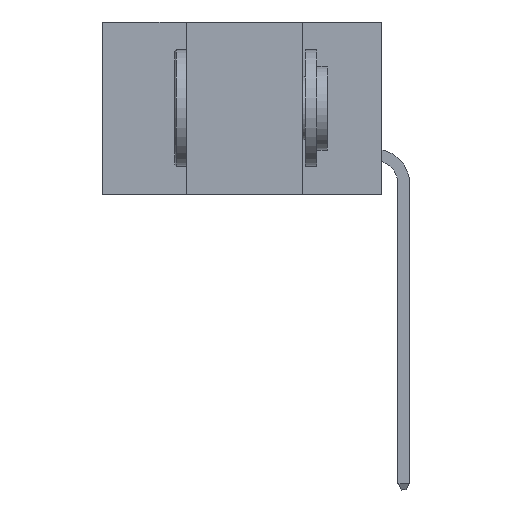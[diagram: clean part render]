
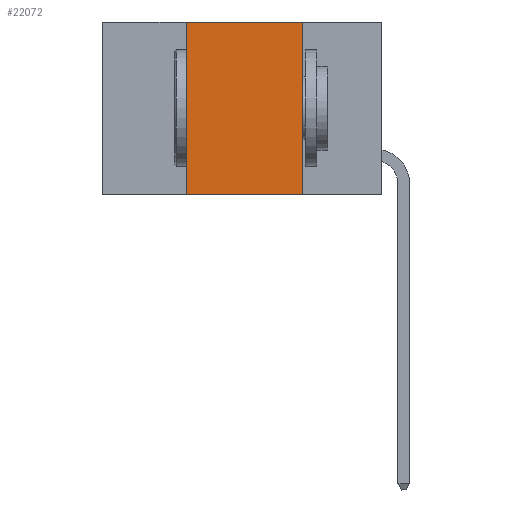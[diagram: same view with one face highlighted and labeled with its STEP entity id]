
A CAD part, left-side view. The second image highlights one B-rep face of the part: STEP entity #22072.
In plain terms, the highlighted planar face has unit normal (-1, 0, 0).
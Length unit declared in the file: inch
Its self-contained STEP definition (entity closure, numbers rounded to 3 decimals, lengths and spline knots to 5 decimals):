
#515 = VECTOR ( 'NONE', #1499, 39.37008 ) ;
#732 = FACE_OUTER_BOUND ( 'NONE', #16419, .T. ) ;
#814 = VERTEX_POINT ( 'NONE', #11368 ) ;
#1448 = ORIENTED_EDGE ( 'NONE', *, *, #7337, .F. ) ;
#1499 = DIRECTION ( 'NONE',  ( 0., 0., 1. ) ) ;
#1758 = CARTESIAN_POINT ( 'NONE',  ( 0., 0.17, 0. ) ) ;
#1856 = VERTEX_POINT ( 'NONE', #5703 ) ;
#3230 = CARTESIAN_POINT ( 'NONE',  ( 0., 0.6, -0.37 ) ) ;
#3730 = PLANE ( 'NONE',  #12339 ) ;
#4260 = VECTOR ( 'NONE', #7290, 39.37008 ) ;
#4717 = VECTOR ( 'NONE', #5380, 39.37008 ) ;
#5380 = DIRECTION ( 'NONE',  ( 0., 0., -1. ) ) ;
#5703 = CARTESIAN_POINT ( 'NONE',  ( 0., 0.17, 0. ) ) ;
#7290 = DIRECTION ( 'NONE',  ( 0., -1., 0. ) ) ;
#7337 = EDGE_CURVE ( 'NONE', #1856, #11195, #24526, .T. ) ;
#9447 = DIRECTION ( 'NONE',  ( 0., -1., 0. ) ) ;
#9757 = DIRECTION ( 'NONE',  ( 0., 0., -1. ) ) ;
#10421 = EDGE_CURVE ( 'NONE', #814, #11195, #19654, .T. ) ;
#10618 = LINE ( 'NONE', #18904, #18927 ) ;
#10801 = ORIENTED_EDGE ( 'NONE', *, *, #20594, .F. ) ;
#11069 = LINE ( 'NONE', #11389, #515 ) ;
#11195 = VERTEX_POINT ( 'NONE', #24838 ) ;
#11368 = CARTESIAN_POINT ( 'NONE',  ( 0., 0.42, -0.37 ) ) ;
#11389 = CARTESIAN_POINT ( 'NONE',  ( 0., 0.42, 0. ) ) ;
#12160 = VERTEX_POINT ( 'NONE', #24221 ) ;
#12339 = AXIS2_PLACEMENT_3D ( 'NONE', #17303, #21103, #9757 ) ;
#16419 = EDGE_LOOP ( 'NONE', ( #1448, #17337, #10801, #18229 ) ) ;
#17303 = CARTESIAN_POINT ( 'NONE',  ( 0., 0.6, 0. ) ) ;
#17337 = ORIENTED_EDGE ( 'NONE', *, *, #18413, .F. ) ;
#18229 = ORIENTED_EDGE ( 'NONE', *, *, #10421, .T. ) ;
#18413 = EDGE_CURVE ( 'NONE', #12160, #1856, #10618, .T. ) ;
#18904 = CARTESIAN_POINT ( 'NONE',  ( 0., 0.6, 0. ) ) ;
#18927 = VECTOR ( 'NONE', #9447, 39.37008 ) ;
#19654 = LINE ( 'NONE', #3230, #4260 ) ;
#20594 = EDGE_CURVE ( 'NONE', #814, #12160, #11069, .T. ) ;
#21103 = DIRECTION ( 'NONE',  ( 1., 0., 0. ) ) ;
#22072 = ADVANCED_FACE ( 'NONE', ( #732 ), #3730, .F. ) ;
#24221 = CARTESIAN_POINT ( 'NONE',  ( 0., 0.42, 0. ) ) ;
#24526 = LINE ( 'NONE', #1758, #4717 ) ;
#24838 = CARTESIAN_POINT ( 'NONE',  ( 0., 0.17, -0.37 ) ) ;
